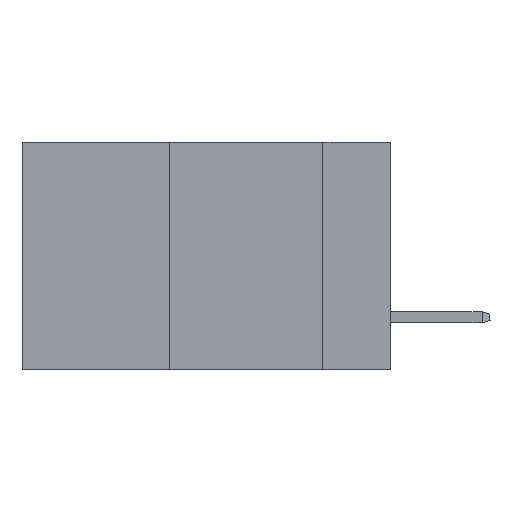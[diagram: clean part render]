
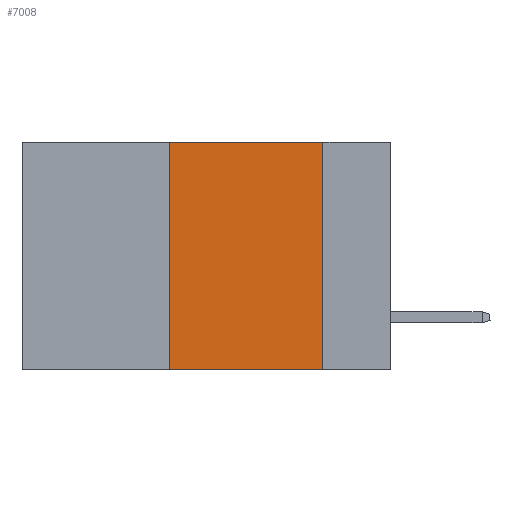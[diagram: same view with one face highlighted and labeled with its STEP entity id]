
A CAD part, left-side view. The second image highlights one B-rep face of the part: STEP entity #7008.
In plain terms, the highlighted planar face has unit normal (-1, 0, 0).
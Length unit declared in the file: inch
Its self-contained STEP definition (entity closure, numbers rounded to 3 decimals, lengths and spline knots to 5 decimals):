
#703 = EDGE_CURVE ( 'NONE', #4800, #19140, #16718, .T. ) ;
#1245 = VECTOR ( 'NONE', #8575, 39.37008 ) ;
#3540 = LINE ( 'NONE', #23760, #3918 ) ;
#3918 = VECTOR ( 'NONE', #28393, 39.37008 ) ;
#4181 = EDGE_CURVE ( 'NONE', #4800, #14598, #3540, .T. ) ;
#4800 = VERTEX_POINT ( 'NONE', #5007 ) ;
#5007 = CARTESIAN_POINT ( 'NONE',  ( 0., 0.36, -0.37 ) ) ;
#5031 = AXIS2_PLACEMENT_3D ( 'NONE', #11022, #21146, #29559 ) ;
#7008 = ADVANCED_FACE ( 'NONE', ( #19079 ), #9003, .F. ) ;
#8575 = DIRECTION ( 'NONE',  ( 0., 0., -1. ) ) ;
#9003 = PLANE ( 'NONE',  #5031 ) ;
#9117 = CARTESIAN_POINT ( 'NONE',  ( 0., 0.6, 0. ) ) ;
#11022 = CARTESIAN_POINT ( 'NONE',  ( 0., 0.6, 0. ) ) ;
#12909 = LINE ( 'NONE', #29264, #1245 ) ;
#14418 = EDGE_LOOP ( 'NONE', ( #25185, #15287, #28757, #21382 ) ) ;
#14598 = VERTEX_POINT ( 'NONE', #22138 ) ;
#15287 = ORIENTED_EDGE ( 'NONE', *, *, #27343, .F. ) ;
#16718 = LINE ( 'NONE', #27579, #21040 ) ;
#17219 = CARTESIAN_POINT ( 'NONE',  ( 0., 0.11, 0. ) ) ;
#17703 = LINE ( 'NONE', #9117, #26667 ) ;
#19079 = FACE_OUTER_BOUND ( 'NONE', #14418, .T. ) ;
#19140 = VERTEX_POINT ( 'NONE', #22418 ) ;
#21040 = VECTOR ( 'NONE', #23078, 39.37008 ) ;
#21146 = DIRECTION ( 'NONE',  ( 1., 0., 0. ) ) ;
#21382 = ORIENTED_EDGE ( 'NONE', *, *, #4181, .T. ) ;
#21779 = VERTEX_POINT ( 'NONE', #17219 ) ;
#22138 = CARTESIAN_POINT ( 'NONE',  ( 0., 0.11, -0.37 ) ) ;
#22418 = CARTESIAN_POINT ( 'NONE',  ( 0., 0.36, 0. ) ) ;
#23078 = DIRECTION ( 'NONE',  ( 0., 0., 1. ) ) ;
#23760 = CARTESIAN_POINT ( 'NONE',  ( 0., 0.6, -0.37 ) ) ;
#25185 = ORIENTED_EDGE ( 'NONE', *, *, #25416, .F. ) ;
#25416 = EDGE_CURVE ( 'NONE', #21779, #14598, #12909, .T. ) ;
#25486 = DIRECTION ( 'NONE',  ( 0., -1., 0. ) ) ;
#26667 = VECTOR ( 'NONE', #25486, 39.37008 ) ;
#27343 = EDGE_CURVE ( 'NONE', #19140, #21779, #17703, .T. ) ;
#27579 = CARTESIAN_POINT ( 'NONE',  ( 0., 0.36, 0. ) ) ;
#28393 = DIRECTION ( 'NONE',  ( 0., -1., 0. ) ) ;
#28757 = ORIENTED_EDGE ( 'NONE', *, *, #703, .F. ) ;
#29264 = CARTESIAN_POINT ( 'NONE',  ( 0., 0.11, 0. ) ) ;
#29559 = DIRECTION ( 'NONE',  ( 0., 0., -1. ) ) ;
